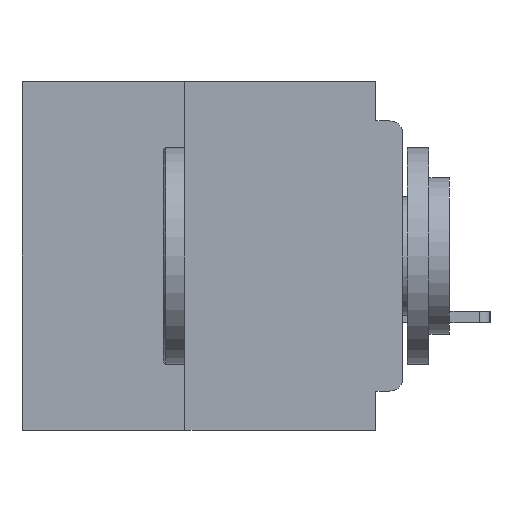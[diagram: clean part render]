
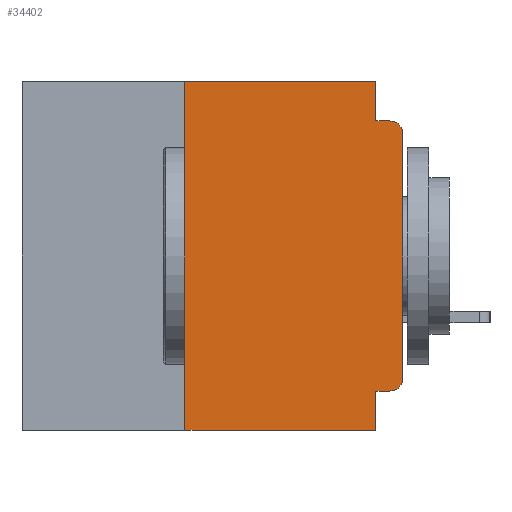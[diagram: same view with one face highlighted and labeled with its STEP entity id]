
A CAD part, left-side view. The second image highlights one B-rep face of the part: STEP entity #34402.
In plain terms, the highlighted planar face has unit normal (-1, 0, 0).
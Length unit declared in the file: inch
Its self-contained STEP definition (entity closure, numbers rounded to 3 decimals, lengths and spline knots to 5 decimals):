
#868 = CARTESIAN_POINT ( 'NONE',  ( 0., 0.015, -0.355 ) ) ;
#2566 = FACE_OUTER_BOUND ( 'NONE', #34760, .T. ) ;
#2655 = CARTESIAN_POINT ( 'NONE',  ( 0., 0.25, -0.4 ) ) ;
#3578 = DIRECTION ( 'NONE',  ( -1., 0., 0. ) ) ;
#4252 = LINE ( 'NONE', #32378, #24973 ) ;
#5538 = CIRCLE ( 'NONE', #8035, 0.015 ) ;
#5698 = DIRECTION ( 'NONE',  ( 0., -1., 0. ) ) ;
#6011 = ORIENTED_EDGE ( 'NONE', *, *, #45909, .F. ) ;
#6027 = CARTESIAN_POINT ( 'NONE',  ( 0., 0., -0.045 ) ) ;
#6463 = EDGE_CURVE ( 'NONE', #19690, #52344, #41544, .T. ) ;
#8035 = AXIS2_PLACEMENT_3D ( 'NONE', #38079, #13473, #42249 ) ;
#8247 = CIRCLE ( 'NONE', #28023, 0.015 ) ;
#8571 = LINE ( 'NONE', #28922, #18322 ) ;
#8573 = CARTESIAN_POINT ( 'NONE',  ( 0., 0.031, -0.4 ) ) ;
#8720 = VECTOR ( 'NONE', #5698, 39.37008 ) ;
#8890 = EDGE_CURVE ( 'NONE', #40613, #12093, #27097, .T. ) ;
#10469 = EDGE_CURVE ( 'NONE', #40748, #24452, #4252, .T. ) ;
#10525 = CARTESIAN_POINT ( 'NONE',  ( 0., 0., 0. ) ) ;
#11934 = DIRECTION ( 'NONE',  ( 0., 0., -1. ) ) ;
#11974 = VERTEX_POINT ( 'NONE', #22776 ) ;
#12093 = VERTEX_POINT ( 'NONE', #27558 ) ;
#12464 = LINE ( 'NONE', #19512, #35619 ) ;
#13108 = ORIENTED_EDGE ( 'NONE', *, *, #10469, .F. ) ;
#13205 = PLANE ( 'NONE',  #29922 ) ;
#13447 = CARTESIAN_POINT ( 'NONE',  ( 0., 0.031, 0. ) ) ;
#13473 = DIRECTION ( 'NONE',  ( -1., 0., 0. ) ) ;
#13879 = ORIENTED_EDGE ( 'NONE', *, *, #21442, .F. ) ;
#14255 = DIRECTION ( 'NONE',  ( 0., -1., 0. ) ) ;
#14408 = CARTESIAN_POINT ( 'NONE',  ( 0., 0.031, -0.045 ) ) ;
#16342 = EDGE_CURVE ( 'NONE', #19690, #11974, #8247, .T. ) ;
#16772 = DIRECTION ( 'NONE',  ( 0., 0., -1. ) ) ;
#17138 = VECTOR ( 'NONE', #26290, 39.37008 ) ;
#17693 = CARTESIAN_POINT ( 'NONE',  ( 0., 0.031, -0.355 ) ) ;
#18322 = VECTOR ( 'NONE', #16772, 39.37008 ) ;
#19316 = ORIENTED_EDGE ( 'NONE', *, *, #6463, .F. ) ;
#19512 = CARTESIAN_POINT ( 'NONE',  ( 0., 0.437, -0.4 ) ) ;
#19690 = VERTEX_POINT ( 'NONE', #868 ) ;
#19753 = LINE ( 'NONE', #26285, #8720 ) ;
#20171 = VECTOR ( 'NONE', #39317, 39.37008 ) ;
#20188 = VERTEX_POINT ( 'NONE', #41359 ) ;
#20412 = DIRECTION ( 'NONE',  ( 0., 0., 1. ) ) ;
#20626 = ORIENTED_EDGE ( 'NONE', *, *, #29220, .T. ) ;
#21442 = EDGE_CURVE ( 'NONE', #24452, #33795, #19753, .T. ) ;
#21509 = DIRECTION ( 'NONE',  ( 0., 0., -1. ) ) ;
#22704 = EDGE_CURVE ( 'NONE', #11974, #20188, #42021, .T. ) ;
#22776 = CARTESIAN_POINT ( 'NONE',  ( 0., 0., -0.34 ) ) ;
#24144 = CARTESIAN_POINT ( 'NONE',  ( 0., 0.031, -0.4 ) ) ;
#24243 = ORIENTED_EDGE ( 'NONE', *, *, #31788, .T. ) ;
#24452 = VERTEX_POINT ( 'NONE', #31873 ) ;
#24973 = VECTOR ( 'NONE', #20412, 39.37008 ) ;
#26108 = CARTESIAN_POINT ( 'NONE',  ( 0., 0., -0.355 ) ) ;
#26285 = CARTESIAN_POINT ( 'NONE',  ( 0., 0.437, 0. ) ) ;
#26290 = DIRECTION ( 'NONE',  ( 0., 1., 0. ) ) ;
#27097 = LINE ( 'NONE', #6027, #36725 ) ;
#27558 = CARTESIAN_POINT ( 'NONE',  ( 0., 0.015, -0.045 ) ) ;
#28023 = AXIS2_PLACEMENT_3D ( 'NONE', #28371, #3578, #32503 ) ;
#28371 = CARTESIAN_POINT ( 'NONE',  ( 0., 0.015, -0.34 ) ) ;
#28922 = CARTESIAN_POINT ( 'NONE',  ( 0., 0.031, 0. ) ) ;
#29220 = EDGE_CURVE ( 'NONE', #40748, #36932, #12464, .T. ) ;
#29922 = AXIS2_PLACEMENT_3D ( 'NONE', #41971, #46154, #21509 ) ;
#31788 = EDGE_CURVE ( 'NONE', #20188, #12093, #5538, .T. ) ;
#31873 = CARTESIAN_POINT ( 'NONE',  ( 0., 0.25, 0. ) ) ;
#32378 = CARTESIAN_POINT ( 'NONE',  ( 0., 0.25, -0.4 ) ) ;
#32503 = DIRECTION ( 'NONE',  ( 0., 0., -1. ) ) ;
#33795 = VERTEX_POINT ( 'NONE', #13447 ) ;
#34402 = ADVANCED_FACE ( 'NONE', ( #2566 ), #13205, .F. ) ;
#34760 = EDGE_LOOP ( 'NONE', ( #37253, #24243, #52230, #6011, #13879, #13108, #20626, #47242, #19316, #39872 ) ) ;
#34933 = VECTOR ( 'NONE', #11934, 39.37008 ) ;
#35619 = VECTOR ( 'NONE', #44133, 39.37008 ) ;
#36222 = EDGE_CURVE ( 'NONE', #52344, #36932, #45953, .T. ) ;
#36725 = VECTOR ( 'NONE', #14255, 39.37008 ) ;
#36932 = VERTEX_POINT ( 'NONE', #8573 ) ;
#37253 = ORIENTED_EDGE ( 'NONE', *, *, #22704, .T. ) ;
#38079 = CARTESIAN_POINT ( 'NONE',  ( 0., 0.015, -0.06 ) ) ;
#39317 = DIRECTION ( 'NONE',  ( 0., 0., 1. ) ) ;
#39872 = ORIENTED_EDGE ( 'NONE', *, *, #16342, .T. ) ;
#40613 = VERTEX_POINT ( 'NONE', #14408 ) ;
#40748 = VERTEX_POINT ( 'NONE', #2655 ) ;
#41359 = CARTESIAN_POINT ( 'NONE',  ( 0., 0., -0.06 ) ) ;
#41544 = LINE ( 'NONE', #26108, #17138 ) ;
#41971 = CARTESIAN_POINT ( 'NONE',  ( 0., 0.437, 0. ) ) ;
#42021 = LINE ( 'NONE', #10525, #20171 ) ;
#42249 = DIRECTION ( 'NONE',  ( 0., 0., -1. ) ) ;
#44133 = DIRECTION ( 'NONE',  ( 0., -1., 0. ) ) ;
#45909 = EDGE_CURVE ( 'NONE', #33795, #40613, #8571, .T. ) ;
#45953 = LINE ( 'NONE', #24144, #34933 ) ;
#46154 = DIRECTION ( 'NONE',  ( 1., 0., 0. ) ) ;
#47242 = ORIENTED_EDGE ( 'NONE', *, *, #36222, .F. ) ;
#52230 = ORIENTED_EDGE ( 'NONE', *, *, #8890, .F. ) ;
#52344 = VERTEX_POINT ( 'NONE', #17693 ) ;
